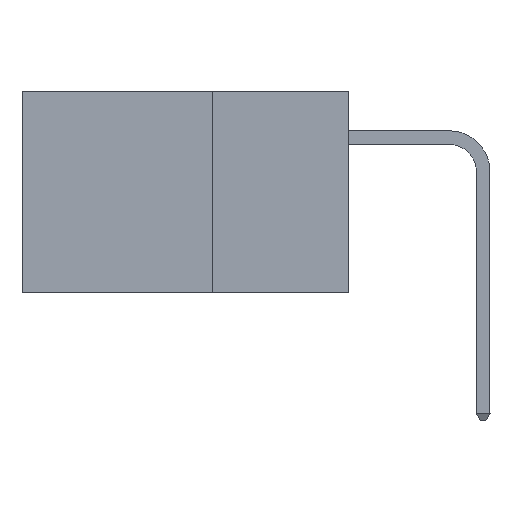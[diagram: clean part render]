
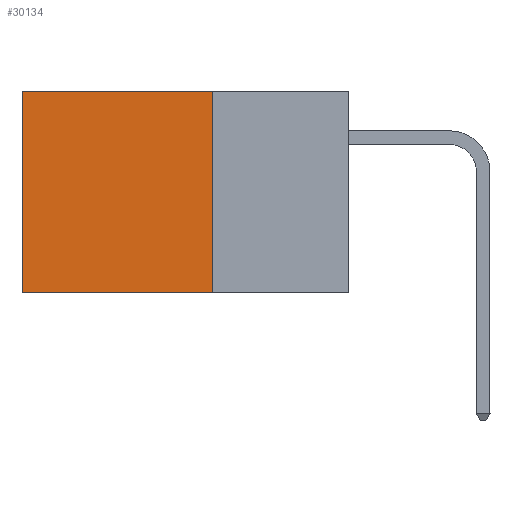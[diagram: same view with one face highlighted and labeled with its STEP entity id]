
A CAD part, left-side view. The second image highlights one B-rep face of the part: STEP entity #30134.
In plain terms, the highlighted planar face has unit normal (-1, 0, 0).
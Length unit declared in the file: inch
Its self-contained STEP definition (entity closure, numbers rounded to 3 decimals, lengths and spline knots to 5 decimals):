
#36 = CARTESIAN_POINT ( 'NONE',  ( 0.2875, 0.25, -0.37 ) ) ;
#1383 = DIRECTION ( 'NONE',  ( 0., 0., -1. ) ) ;
#1774 = CARTESIAN_POINT ( 'NONE',  ( 0.2875, 0.6, -0.37 ) ) ;
#3827 = PLANE ( 'NONE',  #26805 ) ;
#6096 = CARTESIAN_POINT ( 'NONE',  ( 0.2875, 0.25, 0. ) ) ;
#7777 = CARTESIAN_POINT ( 'NONE',  ( 0.2875, 0.6, 0. ) ) ;
#8225 = DIRECTION ( 'NONE',  ( 1., 0., 0. ) ) ;
#9045 = EDGE_CURVE ( 'NONE', #18176, #9597, #23631, .T. ) ;
#9597 = VERTEX_POINT ( 'NONE', #30576 ) ;
#10093 = CARTESIAN_POINT ( 'NONE',  ( 0.2875, 0.25, 0. ) ) ;
#10263 = DIRECTION ( 'NONE',  ( 0., 1., 0. ) ) ;
#10563 = ORIENTED_EDGE ( 'NONE', *, *, #14035, .T. ) ;
#10973 = EDGE_LOOP ( 'NONE', ( #31228, #22863, #16134, #10563 ) ) ;
#10980 = DIRECTION ( 'NONE',  ( 0., 0., -1. ) ) ;
#11135 = CARTESIAN_POINT ( 'NONE',  ( 0.2875, 0.25, 0. ) ) ;
#12300 = VECTOR ( 'NONE', #15029, 39.37008 ) ;
#13179 = LINE ( 'NONE', #18230, #12300 ) ;
#14035 = EDGE_CURVE ( 'NONE', #18176, #14482, #25041, .T. ) ;
#14482 = VERTEX_POINT ( 'NONE', #7777 ) ;
#14821 = DIRECTION ( 'NONE',  ( 0., 1., 0. ) ) ;
#15029 = DIRECTION ( 'NONE',  ( 0., 0., -1. ) ) ;
#16134 = ORIENTED_EDGE ( 'NONE', *, *, #9045, .F. ) ;
#16412 = VECTOR ( 'NONE', #10263, 39.37008 ) ;
#18176 = VERTEX_POINT ( 'NONE', #27984 ) ;
#18230 = CARTESIAN_POINT ( 'NONE',  ( 0.2875, 0.6, 0. ) ) ;
#19859 = LINE ( 'NONE', #36, #29884 ) ;
#22863 = ORIENTED_EDGE ( 'NONE', *, *, #30794, .F. ) ;
#23631 = LINE ( 'NONE', #6096, #27847 ) ;
#24579 = VERTEX_POINT ( 'NONE', #1774 ) ;
#25041 = LINE ( 'NONE', #10093, #16412 ) ;
#26805 = AXIS2_PLACEMENT_3D ( 'NONE', #11135, #8225, #10980 ) ;
#26860 = EDGE_CURVE ( 'NONE', #14482, #24579, #13179, .T. ) ;
#27847 = VECTOR ( 'NONE', #1383, 39.37008 ) ;
#27984 = CARTESIAN_POINT ( 'NONE',  ( 0.2875, 0.25, 0. ) ) ;
#29884 = VECTOR ( 'NONE', #14821, 39.37008 ) ;
#30134 = ADVANCED_FACE ( 'NONE', ( #30651 ), #3827, .F. ) ;
#30576 = CARTESIAN_POINT ( 'NONE',  ( 0.2875, 0.25, -0.37 ) ) ;
#30651 = FACE_OUTER_BOUND ( 'NONE', #10973, .T. ) ;
#30794 = EDGE_CURVE ( 'NONE', #9597, #24579, #19859, .T. ) ;
#31228 = ORIENTED_EDGE ( 'NONE', *, *, #26860, .T. ) ;
